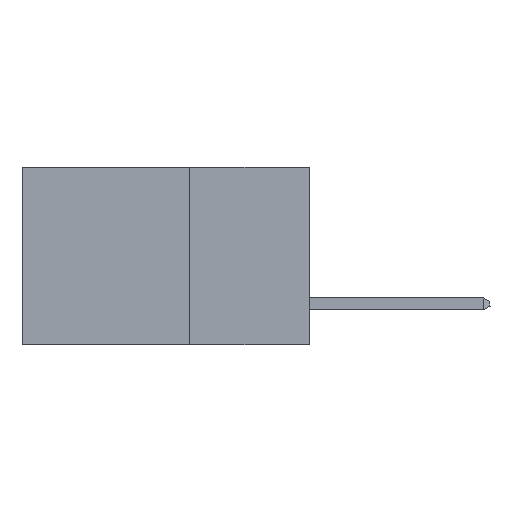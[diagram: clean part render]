
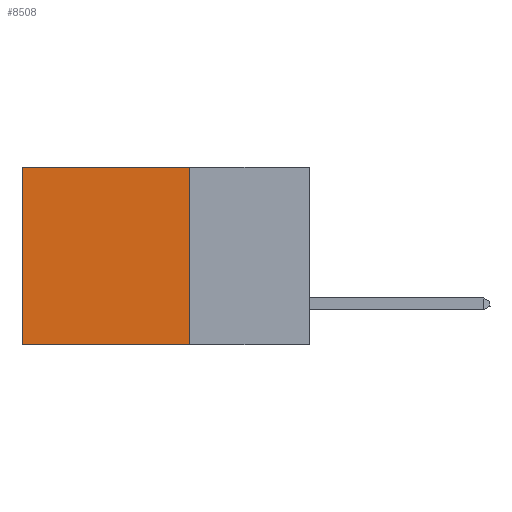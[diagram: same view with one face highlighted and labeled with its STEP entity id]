
A CAD part, left-side view. The second image highlights one B-rep face of the part: STEP entity #8508.
In plain terms, the highlighted planar face has unit normal (-1, 0, 0).
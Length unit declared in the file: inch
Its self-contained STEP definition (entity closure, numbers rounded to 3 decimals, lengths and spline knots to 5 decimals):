
#41 = CARTESIAN_POINT ( 'NONE',  ( 0.2875, 0.6, 0. ) ) ;
#122 = DIRECTION ( 'NONE',  ( 0., 1., 0. ) ) ;
#553 = CARTESIAN_POINT ( 'NONE',  ( 0.2875, 0.25, 0. ) ) ;
#892 = ORIENTED_EDGE ( 'NONE', *, *, #979, .T. ) ;
#979 = EDGE_CURVE ( 'NONE', #3604, #1629, #10074, .T. ) ;
#990 = VECTOR ( 'NONE', #122, 39.37008 ) ;
#1491 = CARTESIAN_POINT ( 'NONE',  ( 0.2875, 0.25, 0. ) ) ;
#1629 = VERTEX_POINT ( 'NONE', #6309 ) ;
#2067 = ORIENTED_EDGE ( 'NONE', *, *, #2228, .F. ) ;
#2140 = DIRECTION ( 'NONE',  ( 0., 0., -1. ) ) ;
#2228 = EDGE_CURVE ( 'NONE', #9444, #1629, #8695, .T. ) ;
#2575 = CARTESIAN_POINT ( 'NONE',  ( 0.2875, 0.25, -0.37 ) ) ;
#2916 = CARTESIAN_POINT ( 'NONE',  ( 0.2875, 0.25, 0. ) ) ;
#3604 = VERTEX_POINT ( 'NONE', #8017 ) ;
#3697 = DIRECTION ( 'NONE',  ( 0., 0., -1. ) ) ;
#4930 = ORIENTED_EDGE ( 'NONE', *, *, #7980, .T. ) ;
#5995 = ORIENTED_EDGE ( 'NONE', *, *, #11046, .F. ) ;
#6309 = CARTESIAN_POINT ( 'NONE',  ( 0.2875, 0.6, -0.37 ) ) ;
#6455 = VECTOR ( 'NONE', #3697, 39.37008 ) ;
#7161 = AXIS2_PLACEMENT_3D ( 'NONE', #10474, #9631, #2140 ) ;
#7438 = EDGE_LOOP ( 'NONE', ( #892, #2067, #5995, #4930 ) ) ;
#7473 = VECTOR ( 'NONE', #8282, 39.37008 ) ;
#7980 = EDGE_CURVE ( 'NONE', #12221, #3604, #8649, .T. ) ;
#8017 = CARTESIAN_POINT ( 'NONE',  ( 0.2875, 0.6, 0. ) ) ;
#8282 = DIRECTION ( 'NONE',  ( 0., 1., 0. ) ) ;
#8508 = ADVANCED_FACE ( 'NONE', ( #12100 ), #10517, .F. ) ;
#8649 = LINE ( 'NONE', #2916, #990 ) ;
#8654 = VECTOR ( 'NONE', #11038, 39.37008 ) ;
#8695 = LINE ( 'NONE', #2575, #7473 ) ;
#9444 = VERTEX_POINT ( 'NONE', #10794 ) ;
#9631 = DIRECTION ( 'NONE',  ( 1., 0., 0. ) ) ;
#10074 = LINE ( 'NONE', #41, #6455 ) ;
#10474 = CARTESIAN_POINT ( 'NONE',  ( 0.2875, 0.25, 0. ) ) ;
#10517 = PLANE ( 'NONE',  #7161 ) ;
#10794 = CARTESIAN_POINT ( 'NONE',  ( 0.2875, 0.25, -0.37 ) ) ;
#11038 = DIRECTION ( 'NONE',  ( 0., 0., -1. ) ) ;
#11046 = EDGE_CURVE ( 'NONE', #12221, #9444, #11505, .T. ) ;
#11505 = LINE ( 'NONE', #553, #8654 ) ;
#12100 = FACE_OUTER_BOUND ( 'NONE', #7438, .T. ) ;
#12221 = VERTEX_POINT ( 'NONE', #1491 ) ;
